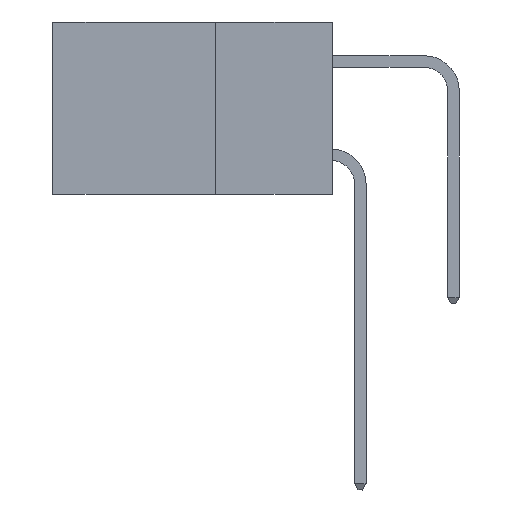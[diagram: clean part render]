
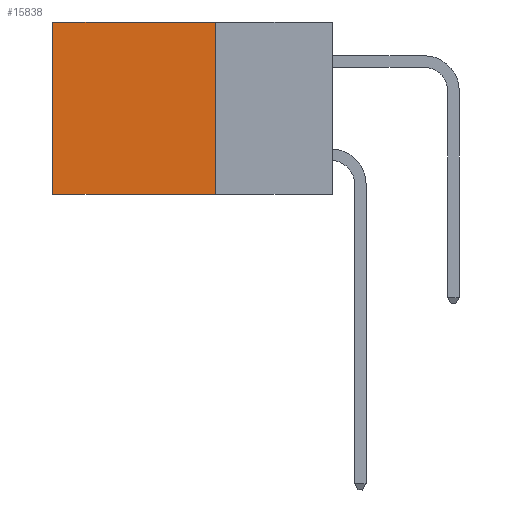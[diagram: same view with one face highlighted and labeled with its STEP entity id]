
A CAD part, left-side view. The second image highlights one B-rep face of the part: STEP entity #15838.
In plain terms, the highlighted planar face has unit normal (-1, 0, 0).
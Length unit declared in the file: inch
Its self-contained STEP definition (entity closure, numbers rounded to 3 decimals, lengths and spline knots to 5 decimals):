
#10 = CARTESIAN_POINT ( 'NONE',  ( 0.298, 0.25, -0.37 ) ) ;
#149 = LINE ( 'NONE', #12394, #11501 ) ;
#1124 = DIRECTION ( 'NONE',  ( 0., 0., -1. ) ) ;
#1133 = LINE ( 'NONE', #21106, #19119 ) ;
#2621 = EDGE_CURVE ( 'NONE', #4780, #16557, #1133, .T. ) ;
#4102 = EDGE_LOOP ( 'NONE', ( #6998, #6410, #12739, #11243 ) ) ;
#4780 = VERTEX_POINT ( 'NONE', #16818 ) ;
#6410 = ORIENTED_EDGE ( 'NONE', *, *, #14776, .F. ) ;
#6998 = ORIENTED_EDGE ( 'NONE', *, *, #26636, .T. ) ;
#7690 = DIRECTION ( 'NONE',  ( 0., 0., -1. ) ) ;
#7844 = CARTESIAN_POINT ( 'NONE',  ( 0.298, 0.25, -0.37 ) ) ;
#8512 = DIRECTION ( 'NONE',  ( 0., 1., 0. ) ) ;
#9108 = VERTEX_POINT ( 'NONE', #20919 ) ;
#9147 = VECTOR ( 'NONE', #21259, 39.37008 ) ;
#10035 = EDGE_CURVE ( 'NONE', #4780, #9108, #25407, .T. ) ;
#10758 = CARTESIAN_POINT ( 'NONE',  ( 0.298, 0.25, 0. ) ) ;
#11243 = ORIENTED_EDGE ( 'NONE', *, *, #10035, .T. ) ;
#11323 = CARTESIAN_POINT ( 'NONE',  ( 0.298, 0.25, 0. ) ) ;
#11501 = VECTOR ( 'NONE', #1124, 39.37008 ) ;
#12197 = FACE_OUTER_BOUND ( 'NONE', #4102, .T. ) ;
#12394 = CARTESIAN_POINT ( 'NONE',  ( 0.298, 0.6, 0. ) ) ;
#12739 = ORIENTED_EDGE ( 'NONE', *, *, #2621, .F. ) ;
#13454 = VECTOR ( 'NONE', #8512, 39.37008 ) ;
#13554 = DIRECTION ( 'NONE',  ( 1., 0., 0. ) ) ;
#14776 = EDGE_CURVE ( 'NONE', #16557, #17380, #15782, .T. ) ;
#15782 = LINE ( 'NONE', #7844, #9147 ) ;
#15838 = ADVANCED_FACE ( 'NONE', ( #12197 ), #22504, .F. ) ;
#16557 = VERTEX_POINT ( 'NONE', #10 ) ;
#16818 = CARTESIAN_POINT ( 'NONE',  ( 0.298, 0.25, 0. ) ) ;
#17380 = VERTEX_POINT ( 'NONE', #18429 ) ;
#18429 = CARTESIAN_POINT ( 'NONE',  ( 0.298, 0.6, -0.37 ) ) ;
#18840 = AXIS2_PLACEMENT_3D ( 'NONE', #11323, #13554, #29107 ) ;
#19119 = VECTOR ( 'NONE', #7690, 39.37008 ) ;
#20919 = CARTESIAN_POINT ( 'NONE',  ( 0.298, 0.6, 0. ) ) ;
#21106 = CARTESIAN_POINT ( 'NONE',  ( 0.298, 0.25, 0. ) ) ;
#21259 = DIRECTION ( 'NONE',  ( 0., 1., 0. ) ) ;
#22504 = PLANE ( 'NONE',  #18840 ) ;
#25407 = LINE ( 'NONE', #10758, #13454 ) ;
#26636 = EDGE_CURVE ( 'NONE', #9108, #17380, #149, .T. ) ;
#29107 = DIRECTION ( 'NONE',  ( 0., 0., -1. ) ) ;
